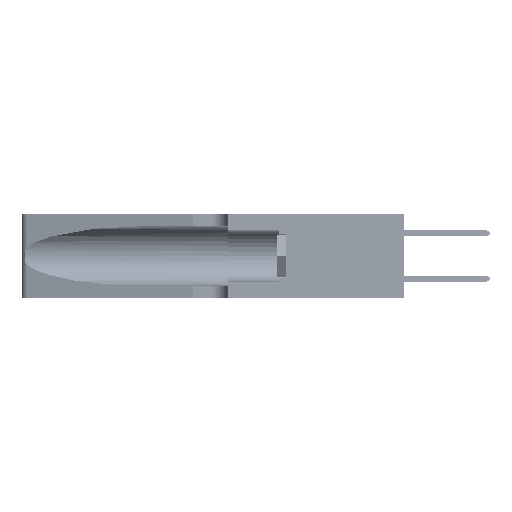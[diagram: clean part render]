
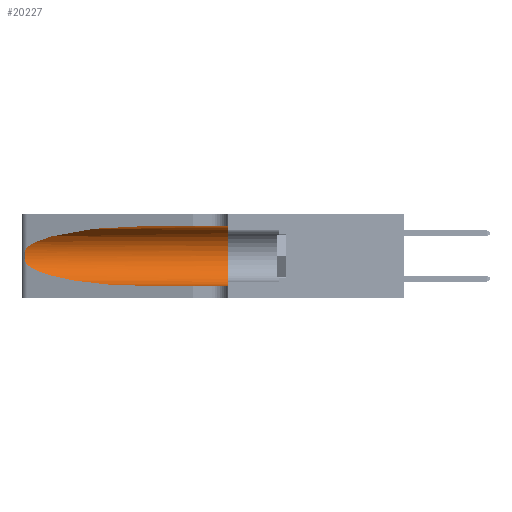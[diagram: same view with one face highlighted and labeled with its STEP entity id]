
A CAD part, left-side view. The second image highlights one B-rep face of the part: STEP entity #20227.
In plain terms, the highlighted cylindrical face has radius 3.308 mm (diameter 6.617 mm), a partial arc.
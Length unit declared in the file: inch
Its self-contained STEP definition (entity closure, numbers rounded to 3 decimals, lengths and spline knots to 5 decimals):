
#874 = EDGE_CURVE ( 'NONE', #46740, #12645, #40168, .T. ) ;
#1593 = VERTEX_POINT ( 'NONE', #48429 ) ;
#2746 = CARTESIAN_POINT ( 'NONE',  ( 0.1305, 1.61858, 0.05475 ) ) ;
#3350 = CARTESIAN_POINT ( 'NONE',  ( 0.25854, 1.2359, 0.20912 ) ) ;
#3951 = CARTESIAN_POINT ( 'NONE',  ( 0.2373, 1.15595, 0.28018 ) ) ;
#6251 = EDGE_CURVE ( 'NONE', #42547, #21563, #35168, .T. ) ;
#7386 = CARTESIAN_POINT ( 'NONE',  ( 0.26075, 1.23896, 0.19203 ) ) ;
#7974 = CARTESIAN_POINT ( 'NONE',  ( 0.18966, 0.96281, 0.31525 ) ) ;
#8720 = ORIENTED_EDGE ( 'NONE', *, *, #47053, .T. ) ;
#9008 =( BOUNDED_CURVE ( )  B_SPLINE_CURVE ( 3, ( #15200, #34758, #19197, #46524 ),
 .UNSPECIFIED., .F., .F. ) 
 B_SPLINE_CURVE_WITH_KNOTS ( ( 4, 4 ),
 ( 3.44316, 4.71239 ),
 .UNSPECIFIED. ) 
 CURVE ( )  GEOMETRIC_REPRESENTATION_ITEM ( )  RATIONAL_B_SPLINE_CURVE ( ( 1., 0.87, 0.87, 1. ) ) 
 REPRESENTATION_ITEM ( '' )  );
#11113 = AXIS2_PLACEMENT_3D ( 'NONE', #14388, #41792, #18368 ) ;
#11307 = LINE ( 'NONE', #2746, #30988 ) ;
#11355 = CARTESIAN_POINT ( 'NONE',  ( 0.26017, 1.23833, 0.17102 ) ) ;
#12073 = DIRECTION ( 'NONE',  ( 0., -1., 0. ) ) ;
#12645 = VERTEX_POINT ( 'NONE', #40506 ) ;
#14143 = EDGE_CURVE ( 'NONE', #46740, #42547, #44359, .T. ) ;
#14388 = CARTESIAN_POINT ( 'NONE',  ( 0.1305, 0.35, 0.185 ) ) ;
#15200 = CARTESIAN_POINT ( 'NONE',  ( 0.25487, 1.22718, 0.14631 ) ) ;
#15334 = CARTESIAN_POINT ( 'NONE',  ( 0.25789, 1.23486, 0.15765 ) ) ;
#15923 = CARTESIAN_POINT ( 'NONE',  ( 0.1305, 0.72297, 0.31525 ) ) ;
#16839 = FACE_OUTER_BOUND ( 'NONE', #33520, .T. ) ;
#17027 = ORIENTED_EDGE ( 'NONE', *, *, #32191, .T. ) ;
#18368 = DIRECTION ( 'NONE',  ( 0., 0., 1. ) ) ;
#19197 = CARTESIAN_POINT ( 'NONE',  ( 0.18966, 0.96281, 0.05475 ) ) ;
#19324 = CARTESIAN_POINT ( 'NONE',  ( 0.25555, 1.22993, 0.14849 ) ) ;
#19674 = EDGE_CURVE ( 'NONE', #28139, #21563, #11307, .T. ) ;
#20227 = ADVANCED_FACE ( 'NONE', ( #16839 ), #46809, .F. ) ;
#20434 = CARTESIAN_POINT ( 'NONE',  ( 0.1305, 0.35, 0.05475 ) ) ;
#20918 = ORIENTED_EDGE ( 'NONE', *, *, #19674, .T. ) ;
#21563 = VERTEX_POINT ( 'NONE', #20434 ) ;
#23273 = CARTESIAN_POINT ( 'NONE',  ( 0.1305, 1.61858, 0.185 ) ) ;
#26569 = CARTESIAN_POINT ( 'NONE',  ( 0.1305, 1.61858, 0.31525 ) ) ;
#27016 = CARTESIAN_POINT ( 'NONE',  ( 0.25787, 1.23484, 0.2124 ) ) ;
#27368 = DIRECTION ( 'NONE',  ( 0., 0., -1. ) ) ;
#28139 = VERTEX_POINT ( 'NONE', #38697 ) ;
#30950 = CARTESIAN_POINT ( 'NONE',  ( 0.26018, 1.23835, 0.19895 ) ) ;
#30988 = VECTOR ( 'NONE', #41984, 39.37008 ) ;
#32191 = EDGE_CURVE ( 'NONE', #1593, #28139, #9008, .T. ) ;
#32358 = CARTESIAN_POINT ( 'NONE',  ( 0.1305, 0.72297, 0.31525 ) ) ;
#32661 = B_SPLINE_CURVE_WITH_KNOTS ( 'NONE', 3,
 ( #46483, #42564, #50382, #27016, #3350, #30950, #7386, #34876, #11355, #38832, #15334, #42733, #19324, #46661 ),
 .UNSPECIFIED., .F., .F.,
 ( 4, 2, 2, 2, 2, 2, 4 ),
 ( 0., 0.00027, 0.00053, 0.00107, 0.0016, 0.00187, 0.00214 ),
 .UNSPECIFIED. ) ;
#32750 = VECTOR ( 'NONE', #38381, 39.37008 ) ;
#33520 = EDGE_LOOP ( 'NONE', ( #35155, #8720, #17027, #20918, #35489, #45605 ) ) ;
#34758 = CARTESIAN_POINT ( 'NONE',  ( 0.2373, 1.15595, 0.08982 ) ) ;
#34876 = CARTESIAN_POINT ( 'NONE',  ( 0.26075, 1.23896, 0.178 ) ) ;
#35155 = ORIENTED_EDGE ( 'NONE', *, *, #874, .T. ) ;
#35168 = CIRCLE ( 'NONE', #11113, 0.13025 ) ;
#35489 = ORIENTED_EDGE ( 'NONE', *, *, #6251, .F. ) ;
#35570 = CARTESIAN_POINT ( 'NONE',  ( 0.1305, 0.35, 0.31525 ) ) ;
#38381 = DIRECTION ( 'NONE',  ( 0., -1., 0. ) ) ;
#38697 = CARTESIAN_POINT ( 'NONE',  ( 0.1305, 0.72297, 0.05475 ) ) ;
#38832 = CARTESIAN_POINT ( 'NONE',  ( 0.25856, 1.23593, 0.16098 ) ) ;
#40168 =( BOUNDED_CURVE ( )  B_SPLINE_CURVE ( 3, ( #15923, #7974, #3951, #43314 ),
 .UNSPECIFIED., .F., .F. ) 
 B_SPLINE_CURVE_WITH_KNOTS ( ( 4, 4 ),
 ( 1.5708, 2.84003 ),
 .UNSPECIFIED. ) 
 CURVE ( )  GEOMETRIC_REPRESENTATION_ITEM ( )  RATIONAL_B_SPLINE_CURVE ( ( 1., 0.87, 0.87, 1. ) ) 
 REPRESENTATION_ITEM ( '' )  );
#40506 = CARTESIAN_POINT ( 'NONE',  ( 0.25487, 1.22718, 0.22369 ) ) ;
#41792 = DIRECTION ( 'NONE',  ( 0., 1., 0. ) ) ;
#41984 = DIRECTION ( 'NONE',  ( 0., -1., 0. ) ) ;
#42547 = VERTEX_POINT ( 'NONE', #35570 ) ;
#42564 = CARTESIAN_POINT ( 'NONE',  ( 0.25555, 1.22994, 0.2215 ) ) ;
#42733 = CARTESIAN_POINT ( 'NONE',  ( 0.25639, 1.23186, 0.15144 ) ) ;
#43314 = CARTESIAN_POINT ( 'NONE',  ( 0.25487, 1.22718, 0.22369 ) ) ;
#44359 = LINE ( 'NONE', #26569, #32750 ) ;
#45605 = ORIENTED_EDGE ( 'NONE', *, *, #14143, .F. ) ;
#46483 = CARTESIAN_POINT ( 'NONE',  ( 0.25487, 1.22718, 0.22369 ) ) ;
#46524 = CARTESIAN_POINT ( 'NONE',  ( 0.1305, 0.72297, 0.05475 ) ) ;
#46661 = CARTESIAN_POINT ( 'NONE',  ( 0.25487, 1.22718, 0.14631 ) ) ;
#46740 = VERTEX_POINT ( 'NONE', #32358 ) ;
#46809 = CYLINDRICAL_SURFACE ( 'NONE', #49576, 0.13025 ) ;
#47053 = EDGE_CURVE ( 'NONE', #12645, #1593, #32661, .T. ) ;
#48429 = CARTESIAN_POINT ( 'NONE',  ( 0.25487, 1.22718, 0.14631 ) ) ;
#49576 = AXIS2_PLACEMENT_3D ( 'NONE', #23273, #12073, #27368 ) ;
#50382 = CARTESIAN_POINT ( 'NONE',  ( 0.25639, 1.23184, 0.21858 ) ) ;
